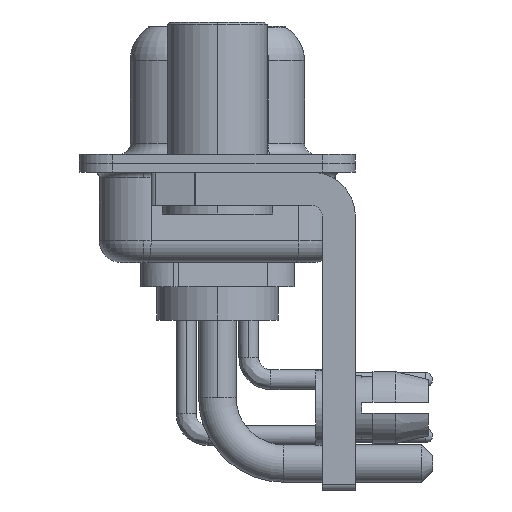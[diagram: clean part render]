
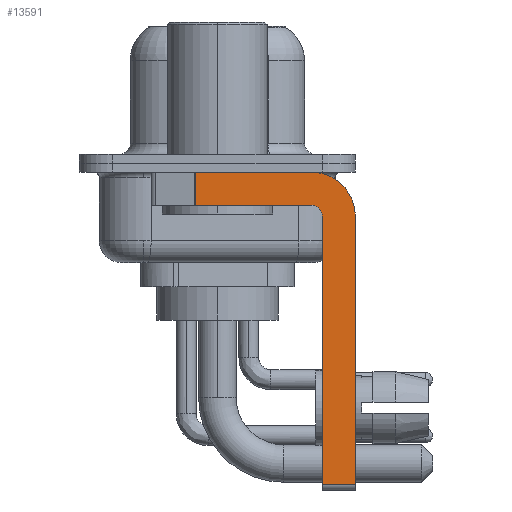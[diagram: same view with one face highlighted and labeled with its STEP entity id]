
A CAD part, left-side view. The second image highlights one B-rep face of the part: STEP entity #13591.
In plain terms, the highlighted planar face has unit normal (-1, 0, 0).
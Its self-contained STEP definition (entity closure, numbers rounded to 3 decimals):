
#427 = DIRECTION ( 'NONE',  ( 0., 0., 1. ) ) ;
#788 = CARTESIAN_POINT ( 'NONE',  ( -2.9, -4.25, -2.4 ) ) ;
#1064 = LINE ( 'NONE', #20154, #23964 ) ;
#1074 = VECTOR ( 'NONE', #20504, 1000. ) ;
#1260 = AXIS2_PLACEMENT_3D ( 'NONE', #19079, #6134, #17215 ) ;
#1812 = DIRECTION ( 'NONE',  ( 0., -1., 0. ) ) ;
#2156 = CARTESIAN_POINT ( 'NONE',  ( -2.9, -4.25, -2.4 ) ) ;
#2257 = ORIENTED_EDGE ( 'NONE', *, *, #19257, .F. ) ;
#2272 = DIRECTION ( 'NONE',  ( -1., 0., 0. ) ) ;
#2281 = CARTESIAN_POINT ( 'NONE',  ( -2.9, -4.25, -14.55 ) ) ;
#2378 = VERTEX_POINT ( 'NONE', #9580 ) ;
#2524 = CARTESIAN_POINT ( 'NONE',  ( -2.9, -4.25, -1.9 ) ) ;
#3383 = VERTEX_POINT ( 'NONE', #18823 ) ;
#3662 = CARTESIAN_POINT ( 'NONE',  ( -2.9, 3., -0.4 ) ) ;
#3886 = LINE ( 'NONE', #22525, #9788 ) ;
#3914 = EDGE_CURVE ( 'NONE', #17742, #21153, #17307, .T. ) ;
#4289 = PLANE ( 'NONE',  #1260 ) ;
#4472 = EDGE_CURVE ( 'NONE', #10090, #3383, #9165, .T. ) ;
#4882 = DIRECTION ( 'NONE',  ( 0., 0., 1. ) ) ;
#5135 = VECTOR ( 'NONE', #24233, 1000. ) ;
#5464 = ORIENTED_EDGE ( 'NONE', *, *, #3914, .T. ) ;
#6134 = DIRECTION ( 'NONE',  ( 1., 0., 0. ) ) ;
#6229 = EDGE_CURVE ( 'NONE', #12129, #21153, #3886, .T. ) ;
#6640 = EDGE_LOOP ( 'NONE', ( #16229, #5464, #22810, #15339, #13367, #13235, #8596, #2257 ) ) ;
#7555 = CARTESIAN_POINT ( 'NONE',  ( -2.9, -6.25, -2.4 ) ) ;
#7666 = CARTESIAN_POINT ( 'NONE',  ( -2.9, -4.75, -2.4 ) ) ;
#8063 = VERTEX_POINT ( 'NONE', #7666 ) ;
#8596 = ORIENTED_EDGE ( 'NONE', *, *, #4472, .F. ) ;
#9165 = LINE ( 'NONE', #7555, #1074 ) ;
#9580 = CARTESIAN_POINT ( 'NONE',  ( -2.9, -4.75, -14.55 ) ) ;
#9788 = VECTOR ( 'NONE', #9896, 1000. ) ;
#9896 = DIRECTION ( 'NONE',  ( 0., 1., 0. ) ) ;
#9942 = FACE_OUTER_BOUND ( 'NONE', #6640, .T. ) ;
#10015 = CARTESIAN_POINT ( 'NONE',  ( -2.9, -4.25, -0.4 ) ) ;
#10090 = VERTEX_POINT ( 'NONE', #18688 ) ;
#10145 = DIRECTION ( 'NONE',  ( 0., 0., -1. ) ) ;
#10660 = EDGE_CURVE ( 'NONE', #8063, #12129, #18837, .T. ) ;
#10980 = AXIS2_PLACEMENT_3D ( 'NONE', #2156, #2272, #427 ) ;
#12129 = VERTEX_POINT ( 'NONE', #2524 ) ;
#12185 = VERTEX_POINT ( 'NONE', #10015 ) ;
#13077 = CARTESIAN_POINT ( 'NONE',  ( -2.9, 0.978, -0.4 ) ) ;
#13235 = ORIENTED_EDGE ( 'NONE', *, *, #20415, .T. ) ;
#13367 = ORIENTED_EDGE ( 'NONE', *, *, #18801, .F. ) ;
#13591 = ADVANCED_FACE ( 'NONE', ( #9942 ), #4289, .F. ) ;
#13599 = DIRECTION ( 'NONE',  ( 1., 0., 0. ) ) ;
#13617 = VECTOR ( 'NONE', #10145, 1000. ) ;
#14737 = LINE ( 'NONE', #3662, #20558 ) ;
#14928 = CIRCLE ( 'NONE', #18084, 2. ) ;
#15339 = ORIENTED_EDGE ( 'NONE', *, *, #10660, .F. ) ;
#15810 = DIRECTION ( 'NONE',  ( 0., 0., -1. ) ) ;
#16229 = ORIENTED_EDGE ( 'NONE', *, *, #23573, .F. ) ;
#17215 = DIRECTION ( 'NONE',  ( 0., 0., -1. ) ) ;
#17307 = LINE ( 'NONE', #19537, #13617 ) ;
#17742 = VERTEX_POINT ( 'NONE', #13077 ) ;
#18084 = AXIS2_PLACEMENT_3D ( 'NONE', #788, #13599, #15810 ) ;
#18688 = CARTESIAN_POINT ( 'NONE',  ( -2.9, -6.25, -2.4 ) ) ;
#18801 = EDGE_CURVE ( 'NONE', #2378, #8063, #1064, .T. ) ;
#18823 = CARTESIAN_POINT ( 'NONE',  ( -2.9, -6.25, -14.55 ) ) ;
#18837 = CIRCLE ( 'NONE', #10980, 0.5 ) ;
#19079 = CARTESIAN_POINT ( 'NONE',  ( -2.9, -4.25, -2.4 ) ) ;
#19153 = LINE ( 'NONE', #2281, #5135 ) ;
#19257 = EDGE_CURVE ( 'NONE', #12185, #10090, #14928, .T. ) ;
#19537 = CARTESIAN_POINT ( 'NONE',  ( -2.9, 0.978, -1.9 ) ) ;
#20154 = CARTESIAN_POINT ( 'NONE',  ( -2.9, -4.75, -14.8 ) ) ;
#20415 = EDGE_CURVE ( 'NONE', #2378, #3383, #19153, .T. ) ;
#20504 = DIRECTION ( 'NONE',  ( 0., 0., -1. ) ) ;
#20558 = VECTOR ( 'NONE', #1812, 1000. ) ;
#21153 = VERTEX_POINT ( 'NONE', #21960 ) ;
#21960 = CARTESIAN_POINT ( 'NONE',  ( -2.9, 0.978, -1.9 ) ) ;
#22525 = CARTESIAN_POINT ( 'NONE',  ( -2.9, -4.25, -1.9 ) ) ;
#22810 = ORIENTED_EDGE ( 'NONE', *, *, #6229, .F. ) ;
#23573 = EDGE_CURVE ( 'NONE', #17742, #12185, #14737, .T. ) ;
#23964 = VECTOR ( 'NONE', #4882, 1000. ) ;
#24233 = DIRECTION ( 'NONE',  ( 0., -1., 0. ) ) ;
